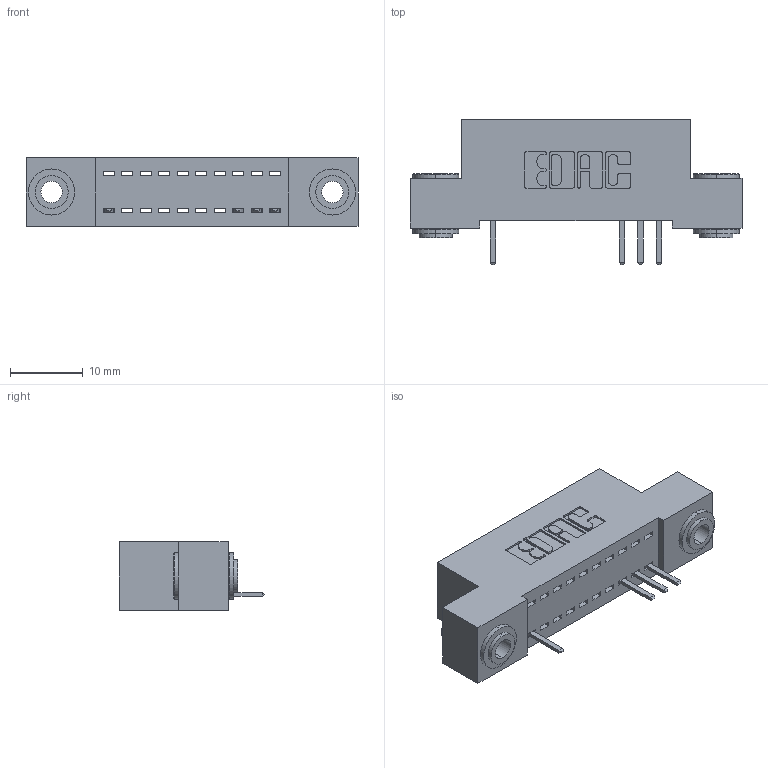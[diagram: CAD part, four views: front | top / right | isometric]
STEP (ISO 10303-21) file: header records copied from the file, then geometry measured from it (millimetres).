
FILE_DESCRIPTION (( 'STEP AP203' ), '1' );
FILE_NAME ('392-010-520-103.STEP', '2018-08-14T20:03:08', ( '' ), ( '' ), 'SwSTEP 2.0', 'SolidWorks 2016', '' );
FILE_SCHEMA (( 'CONFIG_CONTROL_DESIGN' ));
Length unit declared in the file: inch
Products named in the file (4): 392-010-520-103; 342 Part_.156 TH; 345-292-001_345-293-120; 342-250-002_345-250-002-102
Assembly tree (7 placements, depth 2):
  392-010-520-103
    342 Part_.156 TH
    345-292-001_345-293-120  x4
    342-250-002_345-250-002-102  x2
Bounding box: 45.72 x 20.02 x 9.4 mm (x, y, z)
Volume: 3833.6 mm3; surface area: 4865.7 mm2
Topology: 7 solids, 7 shells, 468 faces, 1363 edges, 894 vertices
Faces by surface type: plane 324, cylinder 136, cone 8
Entity records: 10692 total; most frequent: CARTESIAN_POINT 1865, ORIENTED_EDGE 1798, DIRECTION 1653, EDGE_CURVE 899, LINE 743, VECTOR 743, VERTEX_POINT 594, AXIS2_PLACEMENT_3D 455
